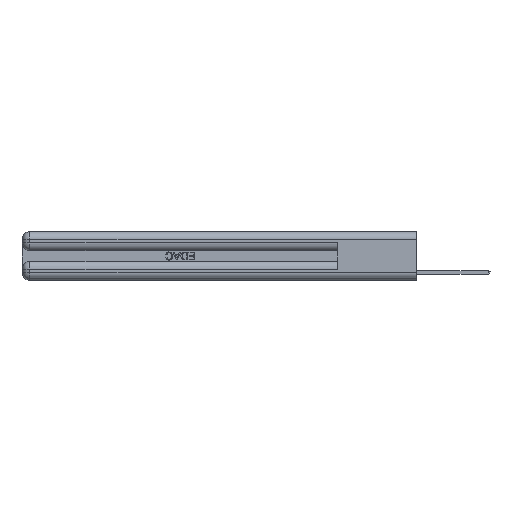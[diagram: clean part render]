
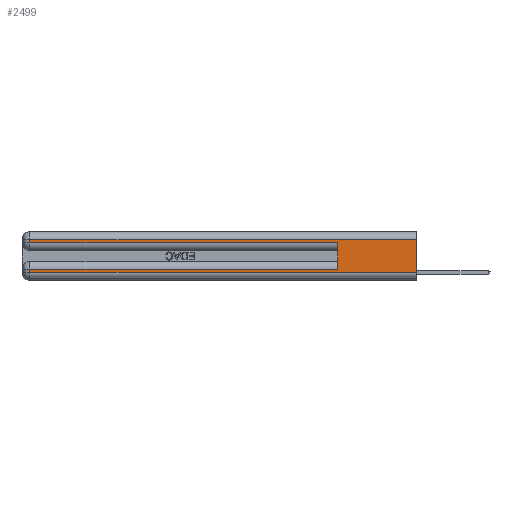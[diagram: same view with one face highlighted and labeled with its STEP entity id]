
A CAD part, left-side view. The second image highlights one B-rep face of the part: STEP entity #2499.
In plain terms, the highlighted planar face has unit normal (-1, 0, 0).
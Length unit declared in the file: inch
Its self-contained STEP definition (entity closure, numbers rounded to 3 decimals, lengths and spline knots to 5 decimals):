
#63 = VERTEX_POINT ( 'NONE', #26850 ) ;
#189 = ORIENTED_EDGE ( 'NONE', *, *, #9462, .F. ) ;
#1276 = DIRECTION ( 'NONE',  ( 0., 0., 1. ) ) ;
#1688 = VERTEX_POINT ( 'NONE', #20907 ) ;
#1714 = CARTESIAN_POINT ( 'NONE',  ( 0., 2.94, 0.37 ) ) ;
#2499 = ADVANCED_FACE ( 'NONE', ( #28289 ), #4931, .F. ) ;
#2567 = DIRECTION ( 'NONE',  ( 0., 0., -1. ) ) ;
#3872 = LINE ( 'NONE', #13612, #10542 ) ;
#4122 = DIRECTION ( 'NONE',  ( 0., 1., 0. ) ) ;
#4931 = PLANE ( 'NONE',  #16746 ) ;
#5098 = CARTESIAN_POINT ( 'NONE',  ( 0., 0., 0.37 ) ) ;
#5438 = ORIENTED_EDGE ( 'NONE', *, *, #20948, .T. ) ;
#7884 = CARTESIAN_POINT ( 'NONE',  ( 0., 2.94, 0.285 ) ) ;
#8119 = VERTEX_POINT ( 'NONE', #28073 ) ;
#8659 = DIRECTION ( 'NONE',  ( 0., 0., -1. ) ) ;
#9275 = VERTEX_POINT ( 'NONE', #26156 ) ;
#9414 = EDGE_LOOP ( 'NONE', ( #11714, #15129, #12789, #24678, #189, #5438, #27353, #21224 ) ) ;
#9462 = EDGE_CURVE ( 'NONE', #63, #9275, #30052, .T. ) ;
#9554 = CARTESIAN_POINT ( 'NONE',  ( 0., 0., 0.31 ) ) ;
#10542 = VECTOR ( 'NONE', #32489, 39.37008 ) ;
#11132 = LINE ( 'NONE', #21697, #20917 ) ;
#11268 = VERTEX_POINT ( 'NONE', #14363 ) ;
#11714 = ORIENTED_EDGE ( 'NONE', *, *, #20296, .F. ) ;
#11863 = CARTESIAN_POINT ( 'NONE',  ( 0., 2.94, 0.06 ) ) ;
#12420 = VECTOR ( 'NONE', #27105, 39.37008 ) ;
#12544 = LINE ( 'NONE', #22942, #33504 ) ;
#12590 = VECTOR ( 'NONE', #8659, 39.37008 ) ;
#12789 = ORIENTED_EDGE ( 'NONE', *, *, #19886, .T. ) ;
#13612 = CARTESIAN_POINT ( 'NONE',  ( 0., 0., 0.31 ) ) ;
#14363 = CARTESIAN_POINT ( 'NONE',  ( 0., 2.94, 0.31 ) ) ;
#15044 = LINE ( 'NONE', #20328, #21321 ) ;
#15129 = ORIENTED_EDGE ( 'NONE', *, *, #26756, .T. ) ;
#16746 = AXIS2_PLACEMENT_3D ( 'NONE', #5098, #20795, #2567 ) ;
#16836 = LINE ( 'NONE', #29607, #12590 ) ;
#17016 = VERTEX_POINT ( 'NONE', #9554 ) ;
#18030 = VERTEX_POINT ( 'NONE', #7884 ) ;
#19121 = VECTOR ( 'NONE', #25713, 39.37008 ) ;
#19144 = DIRECTION ( 'NONE',  ( 0., -1., 0. ) ) ;
#19783 = VECTOR ( 'NONE', #1276, 39.37008 ) ;
#19886 = EDGE_CURVE ( 'NONE', #11268, #18030, #22997, .T. ) ;
#20020 = CARTESIAN_POINT ( 'NONE',  ( 0., 0.6, 0.145 ) ) ;
#20296 = EDGE_CURVE ( 'NONE', #17016, #1688, #16836, .T. ) ;
#20328 = CARTESIAN_POINT ( 'NONE',  ( 0., 0., 0.085 ) ) ;
#20795 = DIRECTION ( 'NONE',  ( 1., 0., 0. ) ) ;
#20907 = CARTESIAN_POINT ( 'NONE',  ( 0., 0., 0.06 ) ) ;
#20917 = VECTOR ( 'NONE', #19144, 39.37008 ) ;
#20948 = EDGE_CURVE ( 'NONE', #63, #8119, #15044, .T. ) ;
#21224 = ORIENTED_EDGE ( 'NONE', *, *, #29206, .T. ) ;
#21321 = VECTOR ( 'NONE', #4122, 39.37008 ) ;
#21697 = CARTESIAN_POINT ( 'NONE',  ( 0., 0., 0.285 ) ) ;
#21847 = CARTESIAN_POINT ( 'NONE',  ( 0., 2.94, 0.37 ) ) ;
#22942 = CARTESIAN_POINT ( 'NONE',  ( 0., 0., 0.06 ) ) ;
#22997 = LINE ( 'NONE', #1714, #19121 ) ;
#24678 = ORIENTED_EDGE ( 'NONE', *, *, #27541, .T. ) ;
#25713 = DIRECTION ( 'NONE',  ( 0., 0., -1. ) ) ;
#26156 = CARTESIAN_POINT ( 'NONE',  ( 0., 0.6, 0.285 ) ) ;
#26756 = EDGE_CURVE ( 'NONE', #17016, #11268, #3872, .T. ) ;
#26850 = CARTESIAN_POINT ( 'NONE',  ( 0., 0.6, 0.085 ) ) ;
#27105 = DIRECTION ( 'NONE',  ( 0., 0., -1. ) ) ;
#27353 = ORIENTED_EDGE ( 'NONE', *, *, #32239, .T. ) ;
#27541 = EDGE_CURVE ( 'NONE', #18030, #9275, #11132, .T. ) ;
#28073 = CARTESIAN_POINT ( 'NONE',  ( 0., 2.94, 0.085 ) ) ;
#28289 = FACE_OUTER_BOUND ( 'NONE', #9414, .T. ) ;
#29000 = VERTEX_POINT ( 'NONE', #11863 ) ;
#29206 = EDGE_CURVE ( 'NONE', #29000, #1688, #12544, .T. ) ;
#29607 = CARTESIAN_POINT ( 'NONE',  ( 0., 0., 0.37 ) ) ;
#30052 = LINE ( 'NONE', #20020, #19783 ) ;
#32239 = EDGE_CURVE ( 'NONE', #8119, #29000, #32556, .T. ) ;
#32489 = DIRECTION ( 'NONE',  ( 0., 1., 0. ) ) ;
#32556 = LINE ( 'NONE', #21847, #12420 ) ;
#33328 = DIRECTION ( 'NONE',  ( 0., -1., 0. ) ) ;
#33504 = VECTOR ( 'NONE', #33328, 39.37008 ) ;
